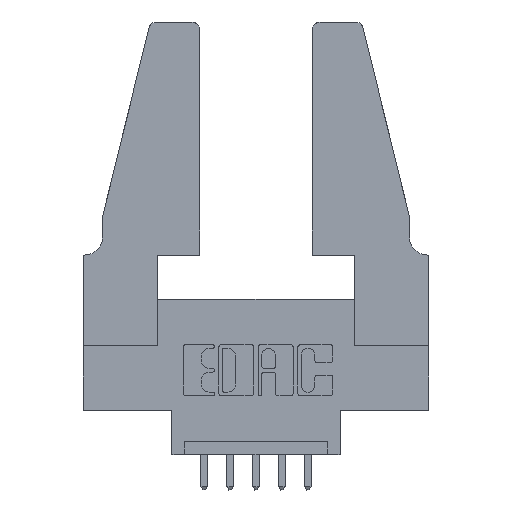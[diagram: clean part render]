
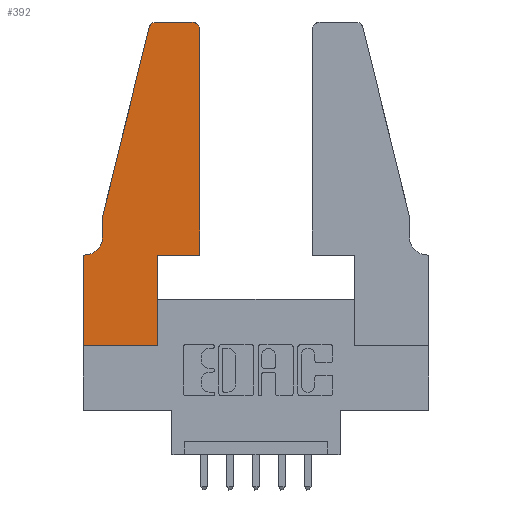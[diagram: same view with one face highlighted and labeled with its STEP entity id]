
A CAD part, top view. The second image highlights one B-rep face of the part: STEP entity #392.
In plain terms, the highlighted planar face has unit normal (0, 0, 1).
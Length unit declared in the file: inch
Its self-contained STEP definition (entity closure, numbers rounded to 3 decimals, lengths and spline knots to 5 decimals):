
#177 = EDGE_CURVE ( 'NONE', #4188, #1880, #607, .T. ) ;
#308 = EDGE_CURVE ( 'NONE', #7112, #10266, #3299, .T. ) ;
#392 = ADVANCED_FACE ( 'NONE', ( #1579 ), #1094, .T. ) ;
#419 = ORIENTED_EDGE ( 'NONE', *, *, #3739, .T. ) ;
#440 = DIRECTION ( 'NONE',  ( 0., 0., 1. ) ) ;
#607 = CIRCLE ( 'NONE', #5983, 0.03 ) ;
#655 = DIRECTION ( 'NONE',  ( 0., -1., 0. ) ) ;
#876 = ORIENTED_EDGE ( 'NONE', *, *, #8098, .T. ) ;
#895 = LINE ( 'NONE', #1470, #8615 ) ;
#1094 = PLANE ( 'NONE',  #2349 ) ;
#1303 = CARTESIAN_POINT ( 'NONE',  ( 0.4205, 1.25, 0.37 ) ) ;
#1470 = CARTESIAN_POINT ( 'NONE',  ( 0.4505, 0.35, 0.37 ) ) ;
#1579 = FACE_OUTER_BOUND ( 'NONE', #10075, .T. ) ;
#1628 = CARTESIAN_POINT ( 'NONE',  ( 0.0755, 0.5, 0.37 ) ) ;
#1701 = DIRECTION ( 'NONE',  ( 1., 0., 0. ) ) ;
#1770 = LINE ( 'NONE', #3040, #3492 ) ;
#1880 = VERTEX_POINT ( 'NONE', #5908 ) ;
#1884 = VECTOR ( 'NONE', #2048, 39.37008 ) ;
#1905 = CARTESIAN_POINT ( 'NONE',  ( 0.4505, 1.22, 0.37 ) ) ;
#1916 = LINE ( 'NONE', #4596, #5532 ) ;
#1926 = EDGE_CURVE ( 'NONE', #3237, #3670, #3003, .T. ) ;
#2048 = DIRECTION ( 'NONE',  ( 1., 0., 0. ) ) ;
#2110 = DIRECTION ( 'NONE',  ( 1., 0., 0. ) ) ;
#2129 = CARTESIAN_POINT ( 'NONE',  ( 0.2865, 0., 0.37 ) ) ;
#2214 = DIRECTION ( 'NONE',  ( -1., 0., 0. ) ) ;
#2312 = CARTESIAN_POINT ( 'NONE',  ( 0.0055, 0.35, 0.37 ) ) ;
#2325 = ORIENTED_EDGE ( 'NONE', *, *, #2530, .T. ) ;
#2349 = AXIS2_PLACEMENT_3D ( 'NONE', #7184, #440, #2110 ) ;
#2360 = CARTESIAN_POINT ( 'NONE',  ( 0., 0., 0.37 ) ) ;
#2513 = CARTESIAN_POINT ( 'NONE',  ( 0.284, 1.22, 0.37 ) ) ;
#2530 = EDGE_CURVE ( 'NONE', #8528, #4188, #7753, .T. ) ;
#2585 = VERTEX_POINT ( 'NONE', #7567 ) ;
#2618 = CARTESIAN_POINT ( 'NONE',  ( 0.0055, 0.42, 0.37 ) ) ;
#2681 = LINE ( 'NONE', #9929, #6127 ) ;
#2781 = CARTESIAN_POINT ( 'NONE',  ( 0., 0., 0.37 ) ) ;
#2938 = VERTEX_POINT ( 'NONE', #1905 ) ;
#3003 = LINE ( 'NONE', #1628, #6567 ) ;
#3040 = CARTESIAN_POINT ( 'NONE',  ( 0.4505, 0.35, 0.37 ) ) ;
#3237 = VERTEX_POINT ( 'NONE', #5448 ) ;
#3299 = LINE ( 'NONE', #6198, #5331 ) ;
#3492 = VECTOR ( 'NONE', #3892, 39.37008 ) ;
#3670 = VERTEX_POINT ( 'NONE', #6930 ) ;
#3739 = EDGE_CURVE ( 'NONE', #8517, #6437, #1916, .T. ) ;
#3787 = DIRECTION ( 'NONE',  ( 0., 1., 0. ) ) ;
#3829 = EDGE_CURVE ( 'NONE', #2585, #2938, #1770, .T. ) ;
#3892 = DIRECTION ( 'NONE',  ( 0., 1., 0. ) ) ;
#4126 = AXIS2_PLACEMENT_3D ( 'NONE', #10239, #9420, #1701 ) ;
#4188 = VERTEX_POINT ( 'NONE', #8425 ) ;
#4448 = CARTESIAN_POINT ( 'NONE',  ( 0., 0., 0.37 ) ) ;
#4538 = VECTOR ( 'NONE', #655, 39.37008 ) ;
#4596 = CARTESIAN_POINT ( 'NONE',  ( 0.2865, 0.35, 0.37 ) ) ;
#4799 = ORIENTED_EDGE ( 'NONE', *, *, #7826, .T. ) ;
#5142 = EDGE_CURVE ( 'NONE', #1880, #3237, #2681, .T. ) ;
#5182 = ORIENTED_EDGE ( 'NONE', *, *, #5142, .T. ) ;
#5331 = VECTOR ( 'NONE', #7033, 39.37008 ) ;
#5448 = CARTESIAN_POINT ( 'NONE',  ( 0.0755, 0.5, 0.37 ) ) ;
#5532 = VECTOR ( 'NONE', #3787, 39.37008 ) ;
#5676 = DIRECTION ( 'NONE',  ( -0.239, -0.971, 0. ) ) ;
#5813 = DIRECTION ( 'NONE',  ( 0., -1., 0. ) ) ;
#5908 = CARTESIAN_POINT ( 'NONE',  ( 0.25487, 1.22718, 0.37 ) ) ;
#5931 = ORIENTED_EDGE ( 'NONE', *, *, #3829, .T. ) ;
#5972 = EDGE_CURVE ( 'NONE', #6967, #8517, #7845, .T. ) ;
#5983 = AXIS2_PLACEMENT_3D ( 'NONE', #2513, #9464, #8455 ) ;
#6110 = LINE ( 'NONE', #2360, #4538 ) ;
#6127 = VECTOR ( 'NONE', #5676, 39.37008 ) ;
#6198 = CARTESIAN_POINT ( 'NONE',  ( 0.0755, 0.35, 0.37 ) ) ;
#6247 = ORIENTED_EDGE ( 'NONE', *, *, #6872, .T. ) ;
#6437 = VERTEX_POINT ( 'NONE', #7783 ) ;
#6567 = VECTOR ( 'NONE', #5813, 39.37008 ) ;
#6872 = EDGE_CURVE ( 'NONE', #3670, #7112, #8625, .T. ) ;
#6930 = CARTESIAN_POINT ( 'NONE',  ( 0.0755, 0.42, 0.37 ) ) ;
#6967 = VERTEX_POINT ( 'NONE', #4448 ) ;
#7033 = DIRECTION ( 'NONE',  ( -1., 0., 0. ) ) ;
#7112 = VERTEX_POINT ( 'NONE', #2312 ) ;
#7184 = CARTESIAN_POINT ( 'NONE',  ( 0., 0.35, 0.37 ) ) ;
#7281 = CARTESIAN_POINT ( 'NONE',  ( 0.2605, 1.25, 0.37 ) ) ;
#7370 = CIRCLE ( 'NONE', #4126, 0.03 ) ;
#7567 = CARTESIAN_POINT ( 'NONE',  ( 0.4505, 0.35, 0.37 ) ) ;
#7753 = LINE ( 'NONE', #7281, #9628 ) ;
#7783 = CARTESIAN_POINT ( 'NONE',  ( 0.2865, 0.35, 0.37 ) ) ;
#7826 = EDGE_CURVE ( 'NONE', #10266, #6967, #6110, .T. ) ;
#7845 = LINE ( 'NONE', #2781, #1884 ) ;
#7901 = ORIENTED_EDGE ( 'NONE', *, *, #308, .T. ) ;
#8098 = EDGE_CURVE ( 'NONE', #6437, #2585, #895, .T. ) ;
#8140 = CARTESIAN_POINT ( 'NONE',  ( 0., 0.35, 0.37 ) ) ;
#8247 = ORIENTED_EDGE ( 'NONE', *, *, #1926, .T. ) ;
#8425 = CARTESIAN_POINT ( 'NONE',  ( 0.284, 1.25, 0.37 ) ) ;
#8455 = DIRECTION ( 'NONE',  ( 1., 0., 0. ) ) ;
#8491 = ORIENTED_EDGE ( 'NONE', *, *, #177, .T. ) ;
#8517 = VERTEX_POINT ( 'NONE', #2129 ) ;
#8528 = VERTEX_POINT ( 'NONE', #1303 ) ;
#8579 = DIRECTION ( 'NONE',  ( -1., 0., 0. ) ) ;
#8615 = VECTOR ( 'NONE', #9872, 39.37008 ) ;
#8625 = CIRCLE ( 'NONE', #9808, 0.07 ) ;
#9171 = ORIENTED_EDGE ( 'NONE', *, *, #5972, .T. ) ;
#9408 = DIRECTION ( 'NONE',  ( 0., 0., -1. ) ) ;
#9420 = DIRECTION ( 'NONE',  ( 0., 0., 1. ) ) ;
#9464 = DIRECTION ( 'NONE',  ( 0., 0., 1. ) ) ;
#9628 = VECTOR ( 'NONE', #2214, 39.37008 ) ;
#9808 = AXIS2_PLACEMENT_3D ( 'NONE', #2618, #9408, #8579 ) ;
#9872 = DIRECTION ( 'NONE',  ( 1., 0., 0. ) ) ;
#9929 = CARTESIAN_POINT ( 'NONE',  ( 0.0755, 0.5, 0.37 ) ) ;
#9981 = EDGE_CURVE ( 'NONE', #2938, #8528, #7370, .T. ) ;
#10075 = EDGE_LOOP ( 'NONE', ( #2325, #8491, #5182, #8247, #6247, #7901, #4799, #9171, #419, #876, #5931, #10722 ) ) ;
#10239 = CARTESIAN_POINT ( 'NONE',  ( 0.4205, 1.22, 0.37 ) ) ;
#10266 = VERTEX_POINT ( 'NONE', #8140 ) ;
#10722 = ORIENTED_EDGE ( 'NONE', *, *, #9981, .T. ) ;
